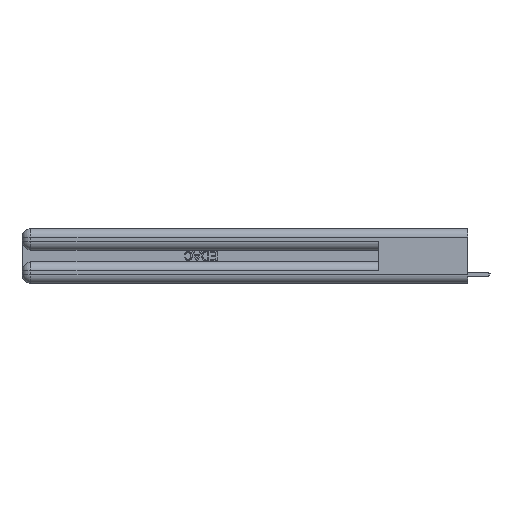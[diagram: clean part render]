
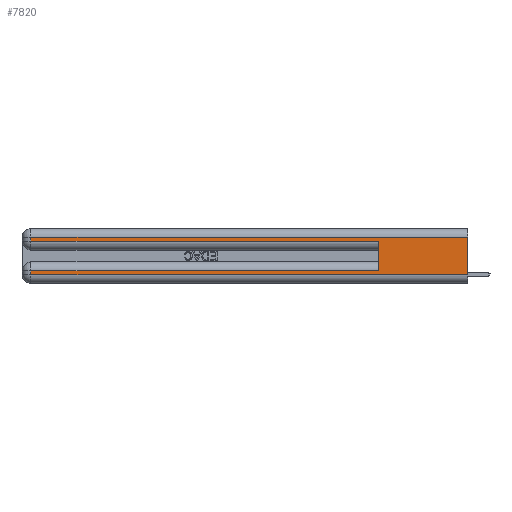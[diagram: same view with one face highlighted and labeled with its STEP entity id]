
A CAD part, left-side view. The second image highlights one B-rep face of the part: STEP entity #7820.
In plain terms, the highlighted planar face has unit normal (-1, 0, 0).
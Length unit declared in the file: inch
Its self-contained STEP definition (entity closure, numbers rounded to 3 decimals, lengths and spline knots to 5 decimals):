
#445 = CARTESIAN_POINT ( 'NONE',  ( 0., 0., 0.06 ) ) ;
#545 = VERTEX_POINT ( 'NONE', #33594 ) ;
#628 = DIRECTION ( 'NONE',  ( 0., -1., 0. ) ) ;
#1350 = CARTESIAN_POINT ( 'NONE',  ( 0., 0., 0.31 ) ) ;
#1456 = EDGE_CURVE ( 'NONE', #10986, #3403, #10993, .T. ) ;
#1654 = VECTOR ( 'NONE', #628, 39.37008 ) ;
#1755 = CARTESIAN_POINT ( 'NONE',  ( 0., 2.94, 0.37 ) ) ;
#1846 = DIRECTION ( 'NONE',  ( 1., 0., 0. ) ) ;
#1909 = ORIENTED_EDGE ( 'NONE', *, *, #22819, .T. ) ;
#2606 = VECTOR ( 'NONE', #10042, 39.37008 ) ;
#3156 = LINE ( 'NONE', #445, #1654 ) ;
#3403 = VERTEX_POINT ( 'NONE', #4374 ) ;
#4187 = FACE_OUTER_BOUND ( 'NONE', #21544, .T. ) ;
#4374 = CARTESIAN_POINT ( 'NONE',  ( 0., 0., 0.06 ) ) ;
#4805 = VECTOR ( 'NONE', #16115, 39.37008 ) ;
#5136 = LINE ( 'NONE', #7843, #4805 ) ;
#5443 = VERTEX_POINT ( 'NONE', #31802 ) ;
#5454 = ORIENTED_EDGE ( 'NONE', *, *, #27549, .T. ) ;
#6931 = VECTOR ( 'NONE', #21828, 39.37008 ) ;
#7367 = EDGE_CURVE ( 'NONE', #34695, #3403, #3156, .T. ) ;
#7475 = VECTOR ( 'NONE', #34497, 39.37008 ) ;
#7820 = ADVANCED_FACE ( 'NONE', ( #4187 ), #12659, .F. ) ;
#7843 = CARTESIAN_POINT ( 'NONE',  ( 0., 0., 0.285 ) ) ;
#8799 = CARTESIAN_POINT ( 'NONE',  ( 0., 2.94, 0.06 ) ) ;
#8929 = ORIENTED_EDGE ( 'NONE', *, *, #1456, .F. ) ;
#9533 = VERTEX_POINT ( 'NONE', #11546 ) ;
#9605 = DIRECTION ( 'NONE',  ( 0., 0., -1. ) ) ;
#9827 = LINE ( 'NONE', #15233, #15520 ) ;
#10042 = DIRECTION ( 'NONE',  ( 0., 0., -1. ) ) ;
#10118 = LINE ( 'NONE', #26868, #21928 ) ;
#10986 = VERTEX_POINT ( 'NONE', #13119 ) ;
#10993 = LINE ( 'NONE', #14419, #6931 ) ;
#11259 = VERTEX_POINT ( 'NONE', #14890 ) ;
#11546 = CARTESIAN_POINT ( 'NONE',  ( 0., 2.94, 0.285 ) ) ;
#12224 = ORIENTED_EDGE ( 'NONE', *, *, #7367, .T. ) ;
#12659 = PLANE ( 'NONE',  #20120 ) ;
#13119 = CARTESIAN_POINT ( 'NONE',  ( 0., 0., 0.31 ) ) ;
#14334 = EDGE_CURVE ( 'NONE', #5443, #20356, #24388, .T. ) ;
#14419 = CARTESIAN_POINT ( 'NONE',  ( 0., 0., 0.37 ) ) ;
#14890 = CARTESIAN_POINT ( 'NONE',  ( 0., 2.94, 0.085 ) ) ;
#15171 = EDGE_CURVE ( 'NONE', #10986, #545, #26051, .T. ) ;
#15219 = EDGE_CURVE ( 'NONE', #5443, #11259, #9827, .T. ) ;
#15233 = CARTESIAN_POINT ( 'NONE',  ( 0., 0., 0.085 ) ) ;
#15520 = VECTOR ( 'NONE', #34669, 39.37008 ) ;
#16115 = DIRECTION ( 'NONE',  ( 0., -1., 0. ) ) ;
#16125 = VECTOR ( 'NONE', #35364, 39.37008 ) ;
#17896 = CARTESIAN_POINT ( 'NONE',  ( 0., 0., 0.37 ) ) ;
#19823 = ORIENTED_EDGE ( 'NONE', *, *, #15219, .T. ) ;
#20120 = AXIS2_PLACEMENT_3D ( 'NONE', #17896, #1846, #9605 ) ;
#20356 = VERTEX_POINT ( 'NONE', #30381 ) ;
#21544 = EDGE_LOOP ( 'NONE', ( #8929, #30197, #5454, #35546, #25901, #19823, #1909, #12224 ) ) ;
#21828 = DIRECTION ( 'NONE',  ( 0., 0., -1. ) ) ;
#21928 = VECTOR ( 'NONE', #32092, 39.37008 ) ;
#22819 = EDGE_CURVE ( 'NONE', #11259, #34695, #10118, .T. ) ;
#24388 = LINE ( 'NONE', #24563, #16125 ) ;
#24563 = CARTESIAN_POINT ( 'NONE',  ( 0., 0.6, 0.145 ) ) ;
#25863 = EDGE_CURVE ( 'NONE', #9533, #20356, #5136, .T. ) ;
#25901 = ORIENTED_EDGE ( 'NONE', *, *, #14334, .F. ) ;
#26051 = LINE ( 'NONE', #1350, #7475 ) ;
#26868 = CARTESIAN_POINT ( 'NONE',  ( 0., 2.94, 0.37 ) ) ;
#27549 = EDGE_CURVE ( 'NONE', #545, #9533, #35406, .T. ) ;
#30197 = ORIENTED_EDGE ( 'NONE', *, *, #15171, .T. ) ;
#30381 = CARTESIAN_POINT ( 'NONE',  ( 0., 0.6, 0.285 ) ) ;
#31802 = CARTESIAN_POINT ( 'NONE',  ( 0., 0.6, 0.085 ) ) ;
#32092 = DIRECTION ( 'NONE',  ( 0., 0., -1. ) ) ;
#33594 = CARTESIAN_POINT ( 'NONE',  ( 0., 2.94, 0.31 ) ) ;
#34497 = DIRECTION ( 'NONE',  ( 0., 1., 0. ) ) ;
#34669 = DIRECTION ( 'NONE',  ( 0., 1., 0. ) ) ;
#34695 = VERTEX_POINT ( 'NONE', #8799 ) ;
#35364 = DIRECTION ( 'NONE',  ( 0., 0., 1. ) ) ;
#35406 = LINE ( 'NONE', #1755, #2606 ) ;
#35546 = ORIENTED_EDGE ( 'NONE', *, *, #25863, .T. ) ;
